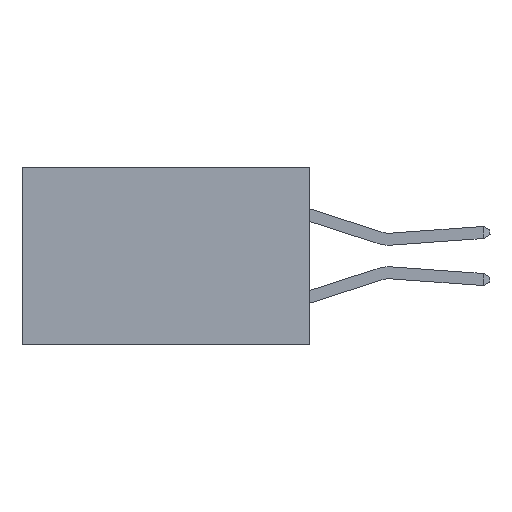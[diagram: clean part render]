
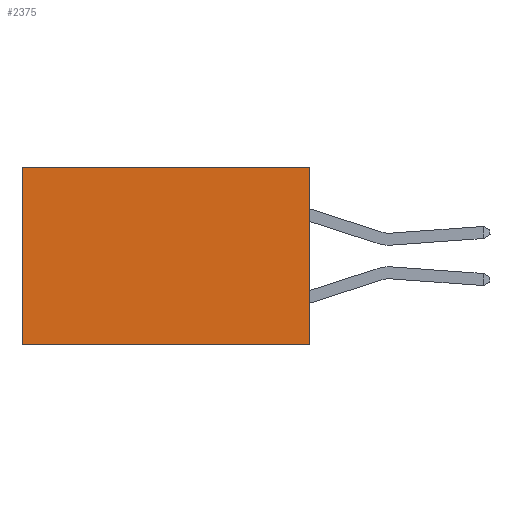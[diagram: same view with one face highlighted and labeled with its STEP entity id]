
A CAD part, left-side view. The second image highlights one B-rep face of the part: STEP entity #2375.
In plain terms, the highlighted planar face has unit normal (-1, 0, 0).
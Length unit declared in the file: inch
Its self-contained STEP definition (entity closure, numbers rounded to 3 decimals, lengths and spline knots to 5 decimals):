
#161 = ORIENTED_EDGE ( 'NONE', *, *, #8401, .F. ) ;
#657 = DIRECTION ( 'NONE',  ( 0., 0., -1. ) ) ;
#1141 = EDGE_CURVE ( 'NONE', #8851, #6556, #10932, .T. ) ;
#1963 = ORIENTED_EDGE ( 'NONE', *, *, #4330, .F. ) ;
#2375 = ADVANCED_FACE ( 'NONE', ( #3572 ), #5261, .F. ) ;
#2498 = LINE ( 'NONE', #7920, #10977 ) ;
#2697 = CARTESIAN_POINT ( 'NONE',  ( 0.2615, 0., 0. ) ) ;
#3572 = FACE_OUTER_BOUND ( 'NONE', #9177, .T. ) ;
#4330 = EDGE_CURVE ( 'NONE', #7191, #11446, #10377, .T. ) ;
#4779 = EDGE_CURVE ( 'NONE', #6556, #11446, #13383, .T. ) ;
#5005 = VECTOR ( 'NONE', #13423, 39.37008 ) ;
#5248 = ORIENTED_EDGE ( 'NONE', *, *, #1141, .T. ) ;
#5261 = PLANE ( 'NONE',  #7049 ) ;
#6556 = VERTEX_POINT ( 'NONE', #9553 ) ;
#7049 = AXIS2_PLACEMENT_3D ( 'NONE', #9659, #13306, #10486 ) ;
#7135 = CARTESIAN_POINT ( 'NONE',  ( 0.2615, 0., 0. ) ) ;
#7152 = CARTESIAN_POINT ( 'NONE',  ( 0.2615, 0., -0.37 ) ) ;
#7191 = VERTEX_POINT ( 'NONE', #7152 ) ;
#7363 = CARTESIAN_POINT ( 'NONE',  ( 0.2615, 0.6, -0.37 ) ) ;
#7871 = DIRECTION ( 'NONE',  ( 0., 0., -1. ) ) ;
#7920 = CARTESIAN_POINT ( 'NONE',  ( 0.2615, 0., -0.37 ) ) ;
#8147 = VECTOR ( 'NONE', #12953, 39.37008 ) ;
#8401 = EDGE_CURVE ( 'NONE', #8851, #7191, #2498, .T. ) ;
#8561 = VECTOR ( 'NONE', #657, 39.37008 ) ;
#8851 = VERTEX_POINT ( 'NONE', #2697 ) ;
#9177 = EDGE_LOOP ( 'NONE', ( #12269, #1963, #161, #5248 ) ) ;
#9553 = CARTESIAN_POINT ( 'NONE',  ( 0.2615, 0.6, 0. ) ) ;
#9659 = CARTESIAN_POINT ( 'NONE',  ( 0.2615, 0., -0.37 ) ) ;
#10377 = LINE ( 'NONE', #13466, #5005 ) ;
#10486 = DIRECTION ( 'NONE',  ( 0., 0., -1. ) ) ;
#10932 = LINE ( 'NONE', #7135, #8147 ) ;
#10977 = VECTOR ( 'NONE', #7871, 39.37008 ) ;
#11446 = VERTEX_POINT ( 'NONE', #7363 ) ;
#11936 = CARTESIAN_POINT ( 'NONE',  ( 0.2615, 0.6, -0.37 ) ) ;
#12269 = ORIENTED_EDGE ( 'NONE', *, *, #4779, .T. ) ;
#12953 = DIRECTION ( 'NONE',  ( 0., 1., 0. ) ) ;
#13306 = DIRECTION ( 'NONE',  ( 1., 0., 0. ) ) ;
#13383 = LINE ( 'NONE', #11936, #8561 ) ;
#13423 = DIRECTION ( 'NONE',  ( 0., 1., 0. ) ) ;
#13466 = CARTESIAN_POINT ( 'NONE',  ( 0.2615, 0., -0.37 ) ) ;
